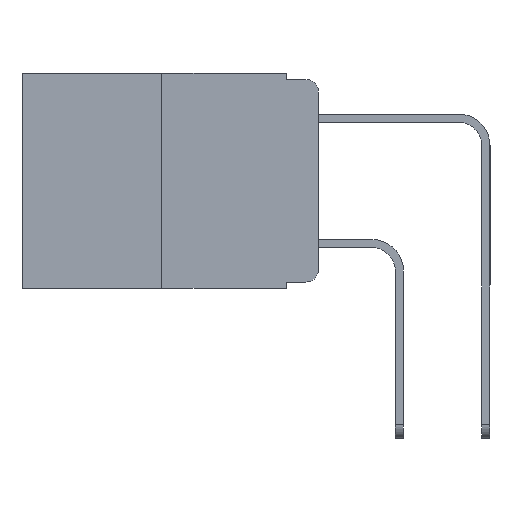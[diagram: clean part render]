
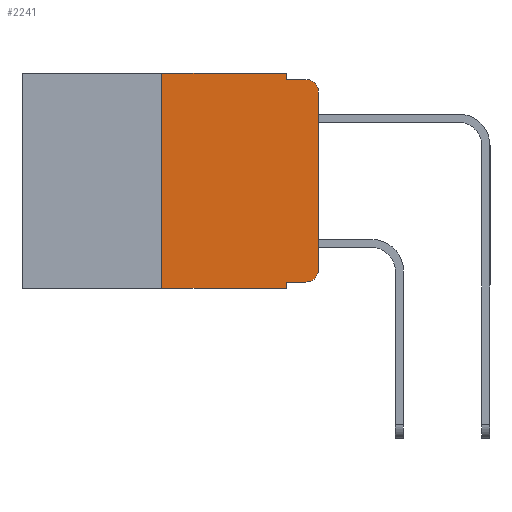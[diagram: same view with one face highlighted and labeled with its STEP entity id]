
A CAD part, left-side view. The second image highlights one B-rep face of the part: STEP entity #2241.
In plain terms, the highlighted planar face has unit normal (-1, 0, 0).
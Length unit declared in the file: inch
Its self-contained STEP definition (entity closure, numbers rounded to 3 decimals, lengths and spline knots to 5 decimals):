
#194 = DIRECTION ( 'NONE',  ( 0., 0., -1. ) ) ;
#259 = CARTESIAN_POINT ( 'NONE',  ( 0., 0.02, -0.313 ) ) ;
#275 = CARTESIAN_POINT ( 'NONE',  ( 0., 0.02, -0.333 ) ) ;
#1131 = CARTESIAN_POINT ( 'NONE',  ( 0., 0.02, -0.01 ) ) ;
#1360 = VERTEX_POINT ( 'NONE', #12612 ) ;
#2241 = ADVANCED_FACE ( 'NONE', ( #8111 ), #9598, .F. ) ;
#3409 = EDGE_CURVE ( 'NONE', #4915, #12431, #15884, .T. ) ;
#3626 = VECTOR ( 'NONE', #11963, 39.37008 ) ;
#3739 = DIRECTION ( 'NONE',  ( 0., 0., 1. ) ) ;
#3851 = VECTOR ( 'NONE', #10257, 39.37008 ) ;
#4222 = EDGE_LOOP ( 'NONE', ( #16077, #7401, #9157, #5827, #8055, #9817, #15051, #11936, #15466, #4891 ) ) ;
#4744 = DIRECTION ( 'NONE',  ( -1., 0., 0. ) ) ;
#4815 = LINE ( 'NONE', #7543, #11859 ) ;
#4891 = ORIENTED_EDGE ( 'NONE', *, *, #3409, .T. ) ;
#4915 = VERTEX_POINT ( 'NONE', #275 ) ;
#5408 = EDGE_CURVE ( 'NONE', #16501, #4915, #8791, .T. ) ;
#5827 = ORIENTED_EDGE ( 'NONE', *, *, #8281, .F. ) ;
#6380 = CARTESIAN_POINT ( 'NONE',  ( 0., 0.473, -0.343 ) ) ;
#6390 = EDGE_CURVE ( 'NONE', #16501, #11130, #7877, .T. ) ;
#6531 = VECTOR ( 'NONE', #9999, 39.37008 ) ;
#7159 = CARTESIAN_POINT ( 'NONE',  ( 0., 0.051, 0. ) ) ;
#7205 = CARTESIAN_POINT ( 'NONE',  ( 0., 0., -0.313 ) ) ;
#7361 = EDGE_CURVE ( 'NONE', #14152, #13678, #17553, .T. ) ;
#7393 = AXIS2_PLACEMENT_3D ( 'NONE', #259, #9388, #194 ) ;
#7401 = ORIENTED_EDGE ( 'NONE', *, *, #10172, .T. ) ;
#7540 = LINE ( 'NONE', #6380, #3626 ) ;
#7543 = CARTESIAN_POINT ( 'NONE',  ( 0., 0.473, 0. ) ) ;
#7750 = LINE ( 'NONE', #8862, #3851 ) ;
#7877 = LINE ( 'NONE', #11356, #6531 ) ;
#7908 = VECTOR ( 'NONE', #14751, 39.37008 ) ;
#8055 = ORIENTED_EDGE ( 'NONE', *, *, #15432, .F. ) ;
#8111 = FACE_OUTER_BOUND ( 'NONE', #4222, .T. ) ;
#8281 = EDGE_CURVE ( 'NONE', #16114, #18104, #14006, .T. ) ;
#8791 = LINE ( 'NONE', #9404, #7908 ) ;
#8862 = CARTESIAN_POINT ( 'NONE',  ( 0., 0., 0. ) ) ;
#8941 = DIRECTION ( 'NONE',  ( 0., -1., 0. ) ) ;
#8980 = CARTESIAN_POINT ( 'NONE',  ( 0., 0.051, -0.343 ) ) ;
#9157 = ORIENTED_EDGE ( 'NONE', *, *, #9240, .F. ) ;
#9233 = DIRECTION ( 'NONE',  ( 0., 0., -1. ) ) ;
#9240 = EDGE_CURVE ( 'NONE', #18104, #10640, #14803, .T. ) ;
#9245 = DIRECTION ( 'NONE',  ( 1., 0., 0. ) ) ;
#9247 = CARTESIAN_POINT ( 'NONE',  ( 0., 0.473, 0. ) ) ;
#9388 = DIRECTION ( 'NONE',  ( -1., 0., 0. ) ) ;
#9404 = CARTESIAN_POINT ( 'NONE',  ( 0., 0.051, -0.333 ) ) ;
#9598 = PLANE ( 'NONE',  #14104 ) ;
#9817 = ORIENTED_EDGE ( 'NONE', *, *, #7361, .F. ) ;
#9999 = DIRECTION ( 'NONE',  ( 0., 0., -1. ) ) ;
#10172 = EDGE_CURVE ( 'NONE', #1360, #10640, #16860, .T. ) ;
#10257 = DIRECTION ( 'NONE',  ( 0., 0., 1. ) ) ;
#10608 = CARTESIAN_POINT ( 'NONE',  ( 0., 0.051, -0.01 ) ) ;
#10640 = VERTEX_POINT ( 'NONE', #1131 ) ;
#11066 = EDGE_CURVE ( 'NONE', #12431, #1360, #7750, .T. ) ;
#11130 = VERTEX_POINT ( 'NONE', #8980 ) ;
#11319 = CARTESIAN_POINT ( 'NONE',  ( 0., 0.051, -0.01 ) ) ;
#11340 = DIRECTION ( 'NONE',  ( 0., 0., -1. ) ) ;
#11356 = CARTESIAN_POINT ( 'NONE',  ( 0., 0.051, 0. ) ) ;
#11859 = VECTOR ( 'NONE', #8941, 39.37008 ) ;
#11936 = ORIENTED_EDGE ( 'NONE', *, *, #6390, .F. ) ;
#11963 = DIRECTION ( 'NONE',  ( 0., -1., 0. ) ) ;
#12213 = CARTESIAN_POINT ( 'NONE',  ( 0., 0.25, 0. ) ) ;
#12431 = VERTEX_POINT ( 'NONE', #7205 ) ;
#12600 = CARTESIAN_POINT ( 'NONE',  ( 0., 0.25, 0. ) ) ;
#12612 = CARTESIAN_POINT ( 'NONE',  ( 0., 0., -0.03 ) ) ;
#12689 = DIRECTION ( 'NONE',  ( 0., -1., 0. ) ) ;
#12787 = CARTESIAN_POINT ( 'NONE',  ( 0., 0.051, -0.333 ) ) ;
#13139 = CARTESIAN_POINT ( 'NONE',  ( 0., 0.02, -0.03 ) ) ;
#13621 = VECTOR ( 'NONE', #3739, 39.37008 ) ;
#13678 = VERTEX_POINT ( 'NONE', #12600 ) ;
#13971 = AXIS2_PLACEMENT_3D ( 'NONE', #13139, #4744, #14459 ) ;
#14006 = LINE ( 'NONE', #7159, #17116 ) ;
#14104 = AXIS2_PLACEMENT_3D ( 'NONE', #9247, #9245, #9233 ) ;
#14152 = VERTEX_POINT ( 'NONE', #16176 ) ;
#14397 = VECTOR ( 'NONE', #12689, 39.37008 ) ;
#14459 = DIRECTION ( 'NONE',  ( 0., 0., -1. ) ) ;
#14644 = CARTESIAN_POINT ( 'NONE',  ( 0., 0.051, 0. ) ) ;
#14751 = DIRECTION ( 'NONE',  ( 0., -1., 0. ) ) ;
#14803 = LINE ( 'NONE', #11319, #14397 ) ;
#15051 = ORIENTED_EDGE ( 'NONE', *, *, #16094, .T. ) ;
#15432 = EDGE_CURVE ( 'NONE', #13678, #16114, #4815, .T. ) ;
#15466 = ORIENTED_EDGE ( 'NONE', *, *, #5408, .T. ) ;
#15884 = CIRCLE ( 'NONE', #7393, 0.02 ) ;
#16077 = ORIENTED_EDGE ( 'NONE', *, *, #11066, .T. ) ;
#16094 = EDGE_CURVE ( 'NONE', #14152, #11130, #7540, .T. ) ;
#16114 = VERTEX_POINT ( 'NONE', #14644 ) ;
#16176 = CARTESIAN_POINT ( 'NONE',  ( 0., 0.25, -0.343 ) ) ;
#16501 = VERTEX_POINT ( 'NONE', #12787 ) ;
#16860 = CIRCLE ( 'NONE', #13971, 0.02 ) ;
#17116 = VECTOR ( 'NONE', #11340, 39.37008 ) ;
#17553 = LINE ( 'NONE', #12213, #13621 ) ;
#18104 = VERTEX_POINT ( 'NONE', #10608 ) ;
